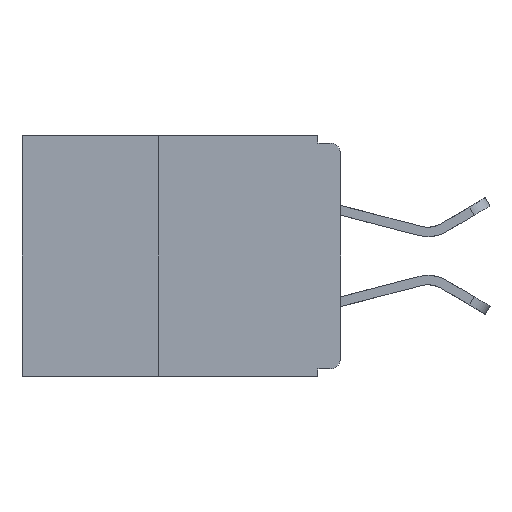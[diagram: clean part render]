
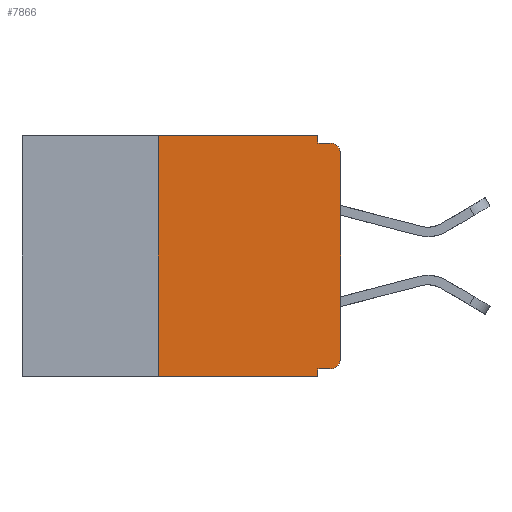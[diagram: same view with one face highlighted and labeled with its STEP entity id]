
A CAD part, left-side view. The second image highlights one B-rep face of the part: STEP entity #7866.
In plain terms, the highlighted planar face has unit normal (-1, 0, 0).
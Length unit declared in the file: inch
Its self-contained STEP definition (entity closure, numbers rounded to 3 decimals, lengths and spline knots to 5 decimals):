
#214 = VECTOR ( 'NONE', #11616, 39.37008 ) ;
#596 = CARTESIAN_POINT ( 'NONE',  ( 0., 0.437, 0. ) ) ;
#792 = DIRECTION ( 'NONE',  ( 0., 0., -1. ) ) ;
#831 = VERTEX_POINT ( 'NONE', #5319 ) ;
#899 = CIRCLE ( 'NONE', #7189, 0.015 ) ;
#918 = DIRECTION ( 'NONE',  ( 0., 0., 1. ) ) ;
#968 = ORIENTED_EDGE ( 'NONE', *, *, #4119, .T. ) ;
#1098 = VERTEX_POINT ( 'NONE', #7976 ) ;
#1116 = CARTESIAN_POINT ( 'NONE',  ( 0., 0.031, 0. ) ) ;
#1270 = LINE ( 'NONE', #8585, #214 ) ;
#1460 = VERTEX_POINT ( 'NONE', #7267 ) ;
#1922 = CARTESIAN_POINT ( 'NONE',  ( 0., 0.437, 0. ) ) ;
#1981 = CARTESIAN_POINT ( 'NONE',  ( 0., 0.031, -0.33 ) ) ;
#2208 = ORIENTED_EDGE ( 'NONE', *, *, #3203, .F. ) ;
#2353 = EDGE_CURVE ( 'NONE', #11421, #1098, #1270, .T. ) ;
#2382 = EDGE_CURVE ( 'NONE', #5393, #7399, #11497, .T. ) ;
#2395 = CIRCLE ( 'NONE', #2679, 0.015 ) ;
#2423 = CARTESIAN_POINT ( 'NONE',  ( 0., 0.031, 0. ) ) ;
#2627 = CARTESIAN_POINT ( 'NONE',  ( 0., 0.015, -0.025 ) ) ;
#2632 = ORIENTED_EDGE ( 'NONE', *, *, #9965, .T. ) ;
#2679 = AXIS2_PLACEMENT_3D ( 'NONE', #2627, #3691, #792 ) ;
#2979 = EDGE_CURVE ( 'NONE', #1098, #5975, #5539, .T. ) ;
#3203 = EDGE_CURVE ( 'NONE', #5975, #1460, #7676, .T. ) ;
#3277 = VERTEX_POINT ( 'NONE', #10094 ) ;
#3337 = ORIENTED_EDGE ( 'NONE', *, *, #2353, .F. ) ;
#3688 = DIRECTION ( 'NONE',  ( 0., 0., -1. ) ) ;
#3691 = DIRECTION ( 'NONE',  ( -1., 0., 0. ) ) ;
#3764 = EDGE_CURVE ( 'NONE', #1460, #7196, #7051, .T. ) ;
#4090 = DIRECTION ( 'NONE',  ( 0., -1., 0. ) ) ;
#4119 = EDGE_CURVE ( 'NONE', #6078, #831, #5359, .T. ) ;
#4138 = DIRECTION ( 'NONE',  ( 0., 0., -1. ) ) ;
#4327 = PLANE ( 'NONE',  #11182 ) ;
#4399 = EDGE_LOOP ( 'NONE', ( #968, #6875, #6093, #2208, #4881, #3337, #2632, #7318, #11822, #4557 ) ) ;
#4557 = ORIENTED_EDGE ( 'NONE', *, *, #7329, .T. ) ;
#4663 = CARTESIAN_POINT ( 'NONE',  ( 0., 0.031, -0.32 ) ) ;
#4874 = DIRECTION ( 'NONE',  ( 0., 0., -1. ) ) ;
#4881 = ORIENTED_EDGE ( 'NONE', *, *, #2979, .F. ) ;
#4921 = DIRECTION ( 'NONE',  ( -1., 0., 0. ) ) ;
#5068 = VECTOR ( 'NONE', #4138, 39.37008 ) ;
#5212 = CARTESIAN_POINT ( 'NONE',  ( 0., 0.437, -0.33 ) ) ;
#5257 = EDGE_CURVE ( 'NONE', #3277, #5393, #7664, .T. ) ;
#5263 = CARTESIAN_POINT ( 'NONE',  ( 0., 0.25, -0.33 ) ) ;
#5319 = CARTESIAN_POINT ( 'NONE',  ( 0., 0., -0.025 ) ) ;
#5359 = LINE ( 'NONE', #9642, #9605 ) ;
#5393 = VERTEX_POINT ( 'NONE', #4663 ) ;
#5539 = LINE ( 'NONE', #1922, #7235 ) ;
#5975 = VERTEX_POINT ( 'NONE', #2423 ) ;
#6020 = VECTOR ( 'NONE', #10193, 39.37008 ) ;
#6078 = VERTEX_POINT ( 'NONE', #8850 ) ;
#6093 = ORIENTED_EDGE ( 'NONE', *, *, #3764, .F. ) ;
#6266 = DIRECTION ( 'NONE',  ( 0., 1., 0. ) ) ;
#6343 = DIRECTION ( 'NONE',  ( 0., 0., -1. ) ) ;
#6689 = CARTESIAN_POINT ( 'NONE',  ( 0., 0.031, -0.33 ) ) ;
#6737 = VECTOR ( 'NONE', #6266, 39.37008 ) ;
#6875 = ORIENTED_EDGE ( 'NONE', *, *, #8505, .T. ) ;
#7051 = LINE ( 'NONE', #11756, #11000 ) ;
#7189 = AXIS2_PLACEMENT_3D ( 'NONE', #9777, #4921, #4874 ) ;
#7196 = VERTEX_POINT ( 'NONE', #10186 ) ;
#7235 = VECTOR ( 'NONE', #7742, 39.37008 ) ;
#7267 = CARTESIAN_POINT ( 'NONE',  ( 0., 0.031, -0.01 ) ) ;
#7318 = ORIENTED_EDGE ( 'NONE', *, *, #2382, .F. ) ;
#7329 = EDGE_CURVE ( 'NONE', #3277, #6078, #899, .T. ) ;
#7334 = CARTESIAN_POINT ( 'NONE',  ( 0., 0., -0.32 ) ) ;
#7399 = VERTEX_POINT ( 'NONE', #1981 ) ;
#7664 = LINE ( 'NONE', #7334, #6737 ) ;
#7676 = LINE ( 'NONE', #1116, #5068 ) ;
#7742 = DIRECTION ( 'NONE',  ( 0., -1., 0. ) ) ;
#7866 = ADVANCED_FACE ( 'NONE', ( #11392 ), #4327, .F. ) ;
#7976 = CARTESIAN_POINT ( 'NONE',  ( 0., 0.25, 0. ) ) ;
#8479 = LINE ( 'NONE', #5212, #6020 ) ;
#8505 = EDGE_CURVE ( 'NONE', #831, #7196, #2395, .T. ) ;
#8585 = CARTESIAN_POINT ( 'NONE',  ( 0., 0.25, -0.33 ) ) ;
#8850 = CARTESIAN_POINT ( 'NONE',  ( 0., 0., -0.305 ) ) ;
#9605 = VECTOR ( 'NONE', #918, 39.37008 ) ;
#9642 = CARTESIAN_POINT ( 'NONE',  ( 0., 0., 0. ) ) ;
#9777 = CARTESIAN_POINT ( 'NONE',  ( 0., 0.015, -0.305 ) ) ;
#9965 = EDGE_CURVE ( 'NONE', #11421, #7399, #8479, .T. ) ;
#10094 = CARTESIAN_POINT ( 'NONE',  ( 0., 0.015, -0.32 ) ) ;
#10186 = CARTESIAN_POINT ( 'NONE',  ( 0., 0.015, -0.01 ) ) ;
#10193 = DIRECTION ( 'NONE',  ( 0., -1., 0. ) ) ;
#10283 = VECTOR ( 'NONE', #3688, 39.37008 ) ;
#11000 = VECTOR ( 'NONE', #4090, 39.37008 ) ;
#11182 = AXIS2_PLACEMENT_3D ( 'NONE', #596, #11260, #6343 ) ;
#11260 = DIRECTION ( 'NONE',  ( 1., 0., 0. ) ) ;
#11392 = FACE_OUTER_BOUND ( 'NONE', #4399, .T. ) ;
#11421 = VERTEX_POINT ( 'NONE', #5263 ) ;
#11497 = LINE ( 'NONE', #6689, #10283 ) ;
#11616 = DIRECTION ( 'NONE',  ( 0., 0., 1. ) ) ;
#11756 = CARTESIAN_POINT ( 'NONE',  ( 0., 0., -0.01 ) ) ;
#11822 = ORIENTED_EDGE ( 'NONE', *, *, #5257, .F. ) ;
